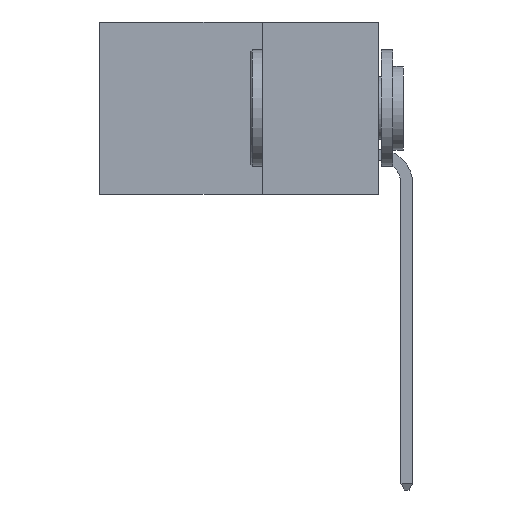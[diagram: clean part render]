
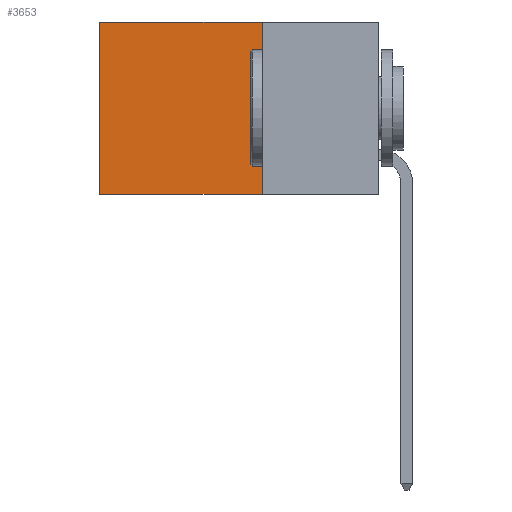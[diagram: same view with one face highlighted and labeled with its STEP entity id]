
A CAD part, left-side view. The second image highlights one B-rep face of the part: STEP entity #3653.
In plain terms, the highlighted planar face has unit normal (-1, 0, 0).
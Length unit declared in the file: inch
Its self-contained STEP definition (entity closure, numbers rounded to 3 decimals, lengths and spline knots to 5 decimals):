
#372 = CARTESIAN_POINT ( 'NONE',  ( 0.2615, 0.6, 0. ) ) ;
#517 = DIRECTION ( 'NONE',  ( 0., 1., 0. ) ) ;
#520 = CARTESIAN_POINT ( 'NONE',  ( 0.2615, 0.25, 0. ) ) ;
#561 = CARTESIAN_POINT ( 'NONE',  ( 0.2615, 0.25, -0.37 ) ) ;
#570 = DIRECTION ( 'NONE',  ( 0., 0., -1. ) ) ;
#1369 = ORIENTED_EDGE ( 'NONE', *, *, #7012, .T. ) ;
#1746 = VECTOR ( 'NONE', #517, 39.37008 ) ;
#1855 = FACE_OUTER_BOUND ( 'NONE', #5762, .T. ) ;
#2045 = ORIENTED_EDGE ( 'NONE', *, *, #7553, .T. ) ;
#2520 = VERTEX_POINT ( 'NONE', #7338 ) ;
#2734 = CARTESIAN_POINT ( 'NONE',  ( 0.2615, 0.6, -0.37 ) ) ;
#3079 = CARTESIAN_POINT ( 'NONE',  ( 0.2615, 0.25, -0.37 ) ) ;
#3653 = ADVANCED_FACE ( 'NONE', ( #1855 ), #5211, .F. ) ;
#3863 = LINE ( 'NONE', #561, #7471 ) ;
#4795 = AXIS2_PLACEMENT_3D ( 'NONE', #5166, #5157, #5144 ) ;
#5077 = DIRECTION ( 'NONE',  ( 0., 0., -1. ) ) ;
#5144 = DIRECTION ( 'NONE',  ( 0., 0., -1. ) ) ;
#5157 = DIRECTION ( 'NONE',  ( 1., 0., 0. ) ) ;
#5166 = CARTESIAN_POINT ( 'NONE',  ( 0.2615, 0.25, -0.37 ) ) ;
#5211 = PLANE ( 'NONE',  #4795 ) ;
#5237 = VERTEX_POINT ( 'NONE', #8620 ) ;
#5521 = VERTEX_POINT ( 'NONE', #7383 ) ;
#5762 = EDGE_LOOP ( 'NONE', ( #2045, #8442, #6859, #1369 ) ) ;
#5865 = VECTOR ( 'NONE', #6232, 39.37008 ) ;
#6232 = DIRECTION ( 'NONE',  ( 0., 1., 0. ) ) ;
#6859 = ORIENTED_EDGE ( 'NONE', *, *, #7016, .F. ) ;
#7012 = EDGE_CURVE ( 'NONE', #2520, #7046, #9597, .T. ) ;
#7015 = VECTOR ( 'NONE', #5077, 39.37008 ) ;
#7016 = EDGE_CURVE ( 'NONE', #2520, #5521, #3863, .T. ) ;
#7046 = VERTEX_POINT ( 'NONE', #372 ) ;
#7338 = CARTESIAN_POINT ( 'NONE',  ( 0.2615, 0.25, 0. ) ) ;
#7383 = CARTESIAN_POINT ( 'NONE',  ( 0.2615, 0.25, -0.37 ) ) ;
#7471 = VECTOR ( 'NONE', #570, 39.37008 ) ;
#7553 = EDGE_CURVE ( 'NONE', #7046, #5237, #8718, .T. ) ;
#7838 = LINE ( 'NONE', #3079, #5865 ) ;
#8442 = ORIENTED_EDGE ( 'NONE', *, *, #9441, .F. ) ;
#8620 = CARTESIAN_POINT ( 'NONE',  ( 0.2615, 0.6, -0.37 ) ) ;
#8718 = LINE ( 'NONE', #2734, #7015 ) ;
#9441 = EDGE_CURVE ( 'NONE', #5521, #5237, #7838, .T. ) ;
#9597 = LINE ( 'NONE', #520, #1746 ) ;
